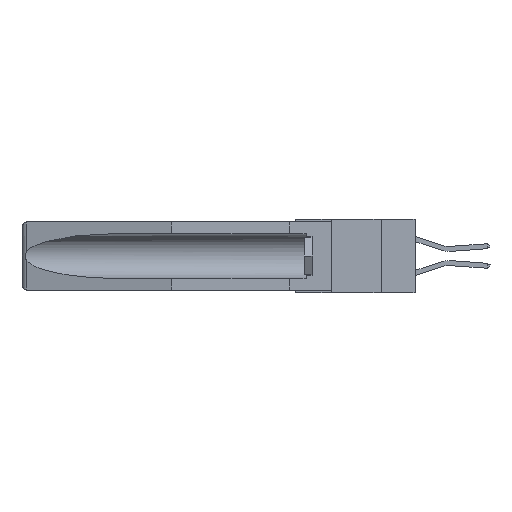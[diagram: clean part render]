
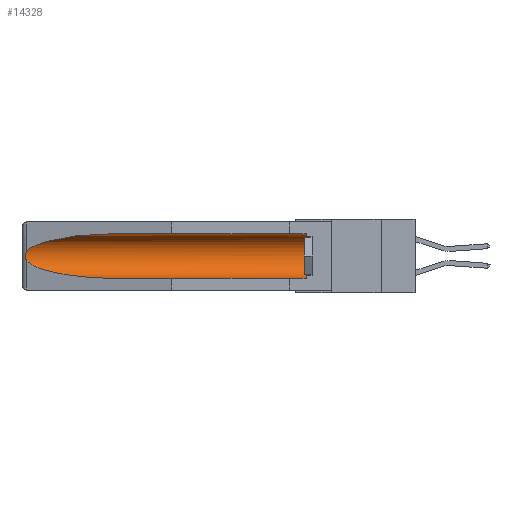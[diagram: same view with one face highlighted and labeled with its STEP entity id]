
A CAD part, left-side view. The second image highlights one B-rep face of the part: STEP entity #14328.
In plain terms, the highlighted cylindrical face has radius 2.857 mm (diameter 5.715 mm), a partial arc.
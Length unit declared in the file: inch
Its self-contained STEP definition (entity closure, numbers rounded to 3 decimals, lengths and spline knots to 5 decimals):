
#73 = B_SPLINE_CURVE_WITH_KNOTS ( 'NONE', 3,
 ( #18737, #18811, #20542, #18667, #11899, #1421, #1572, #13567, #13637, #15088 ),
 .UNSPECIFIED., .F., .F.,
 ( 4, 2, 2, 2, 4 ),
 ( 0., 0.00029, 0.00058, 0.00087, 0.00117 ),
 .UNSPECIFIED. ) ;
#281 = DIRECTION ( 'NONE',  ( 0., -1., 0. ) ) ;
#375 = CARTESIAN_POINT ( 'NONE',  ( 0.155, -0.30754, -0.059 ) ) ;
#984 = ORIENTED_EDGE ( 'NONE', *, *, #20544, .T. ) ;
#1224 = AXIS2_PLACEMENT_3D ( 'NONE', #21011, #281, #10690 ) ;
#1307 = CYLINDRICAL_SURFACE ( 'NONE', #9294, 0.1125 ) ;
#1421 = CARTESIAN_POINT ( 'NONE',  ( 0.2675, 1.53308, -0.17534 ) ) ;
#1572 = CARTESIAN_POINT ( 'NONE',  ( 0.2673, 1.53269, -0.17917 ) ) ;
#1577 = ORIENTED_EDGE ( 'NONE', *, *, #12082, .F. ) ;
#2076 = DIRECTION ( 'NONE',  ( 0., 0., 1. ) ) ;
#2409 = CARTESIAN_POINT ( 'NONE',  ( 0.21114, 1.30732, -0.284 ) ) ;
#3409 = CARTESIAN_POINT ( 'NONE',  ( 0.25451, 1.48313, -0.09465 ) ) ;
#4006 = CIRCLE ( 'NONE', #1224, 0.1125 ) ;
#6884 = EDGE_CURVE ( 'NONE', #11248, #16887, #19540, .T. ) ;
#6887 = CARTESIAN_POINT ( 'NONE',  ( 0.26537, 1.52718, -0.14972 ) ) ;
#6918 = ORIENTED_EDGE ( 'NONE', *, *, #6884, .T. ) ;
#7300 = CARTESIAN_POINT ( 'NONE',  ( 0.155, -0.30754, -0.1715 ) ) ;
#7549 = CARTESIAN_POINT ( 'NONE',  ( 0.155, 1.07973, -0.284 ) ) ;
#7848 = EDGE_LOOP ( 'NONE', ( #19603, #984, #9586, #1577, #12763, #6918 ) ) ;
#9294 = AXIS2_PLACEMENT_3D ( 'NONE', #7300, #10823, #2076 ) ;
#9586 = ORIENTED_EDGE ( 'NONE', *, *, #11202, .T. ) ;
#10166 =( BOUNDED_CURVE ( )  B_SPLINE_CURVE ( 3, ( #19640, #14554, #2409, #7549 ),
 .UNSPECIFIED., .F., .F. ) 
 B_SPLINE_CURVE_WITH_KNOTS ( ( 4, 4 ),
 ( 0.1948, 1.5708 ),
 .UNSPECIFIED. ) 
 CURVE ( )  GEOMETRIC_REPRESENTATION_ITEM ( )  RATIONAL_B_SPLINE_CURVE ( ( 1., 0.848, 0.848, 1. ) ) 
 REPRESENTATION_ITEM ( '' )  );
#10176 = CARTESIAN_POINT ( 'NONE',  ( 0.155, -0.30754, -0.284 ) ) ;
#10690 = DIRECTION ( 'NONE',  ( 0., 0., 1. ) ) ;
#10823 = DIRECTION ( 'NONE',  ( 0., 1., 0. ) ) ;
#10954 = CARTESIAN_POINT ( 'NONE',  ( 0.26537, 1.52718, -0.14972 ) ) ;
#11202 = EDGE_CURVE ( 'NONE', #21206, #16096, #10166, .T. ) ;
#11248 = VERTEX_POINT ( 'NONE', #21609 ) ;
#11439 = VERTEX_POINT ( 'NONE', #14534 ) ;
#11899 = CARTESIAN_POINT ( 'NONE',  ( 0.2675, 1.53308, -0.16763 ) ) ;
#12082 = EDGE_CURVE ( 'NONE', #11439, #16096, #14864, .T. ) ;
#12298 = VECTOR ( 'NONE', #19201, 39.37008 ) ;
#12425 = VECTOR ( 'NONE', #22234, 39.37008 ) ;
#12763 = ORIENTED_EDGE ( 'NONE', *, *, #13799, .T. ) ;
#13567 = CARTESIAN_POINT ( 'NONE',  ( 0.26655, 1.53094, -0.18657 ) ) ;
#13637 = CARTESIAN_POINT ( 'NONE',  ( 0.26597, 1.5296, -0.19026 ) ) ;
#13743 = CARTESIAN_POINT ( 'NONE',  ( 0.21114, 1.30732, -0.059 ) ) ;
#13799 = EDGE_CURVE ( 'NONE', #11439, #11248, #4006, .T. ) ;
#14328 = ADVANCED_FACE ( 'NONE', ( #15078 ), #1307, .F. ) ;
#14534 = CARTESIAN_POINT ( 'NONE',  ( 0.155, 0.126, -0.284 ) ) ;
#14554 = CARTESIAN_POINT ( 'NONE',  ( 0.25451, 1.48313, -0.24835 ) ) ;
#14864 = LINE ( 'NONE', #10176, #12425 ) ;
#15078 = FACE_OUTER_BOUND ( 'NONE', #7848, .T. ) ;
#15088 = CARTESIAN_POINT ( 'NONE',  ( 0.26537, 1.52718, -0.19328 ) ) ;
#15241 = CARTESIAN_POINT ( 'NONE',  ( 0.26537, 1.52718, -0.19328 ) ) ;
#15442 = CARTESIAN_POINT ( 'NONE',  ( 0.155, 1.07973, -0.059 ) ) ;
#16096 = VERTEX_POINT ( 'NONE', #16534 ) ;
#16534 = CARTESIAN_POINT ( 'NONE',  ( 0.155, 1.07973, -0.284 ) ) ;
#16887 = VERTEX_POINT ( 'NONE', #15442 ) ;
#18667 = CARTESIAN_POINT ( 'NONE',  ( 0.2673, 1.5327, -0.16383 ) ) ;
#18737 = CARTESIAN_POINT ( 'NONE',  ( 0.26537, 1.52718, -0.14972 ) ) ;
#18811 = CARTESIAN_POINT ( 'NONE',  ( 0.26597, 1.52961, -0.15275 ) ) ;
#18934 = VERTEX_POINT ( 'NONE', #10954 ) ;
#19201 = DIRECTION ( 'NONE',  ( 0., 1., 0. ) ) ;
#19316 = EDGE_CURVE ( 'NONE', #16887, #18934, #19427, .T. ) ;
#19427 =( BOUNDED_CURVE ( )  B_SPLINE_CURVE ( 3, ( #22308, #13743, #3409, #6887 ),
 .UNSPECIFIED., .F., .T. ) 
 B_SPLINE_CURVE_WITH_KNOTS ( ( 4, 4 ),
 ( 4.71239, 6.08839 ),
 .UNSPECIFIED. ) 
 CURVE ( )  GEOMETRIC_REPRESENTATION_ITEM ( )  RATIONAL_B_SPLINE_CURVE ( ( 1., 0.848, 0.848, 1. ) ) 
 REPRESENTATION_ITEM ( '' )  );
#19540 = LINE ( 'NONE', #375, #12298 ) ;
#19603 = ORIENTED_EDGE ( 'NONE', *, *, #19316, .T. ) ;
#19640 = CARTESIAN_POINT ( 'NONE',  ( 0.26537, 1.52718, -0.19328 ) ) ;
#20542 = CARTESIAN_POINT ( 'NONE',  ( 0.26654, 1.53092, -0.15636 ) ) ;
#20544 = EDGE_CURVE ( 'NONE', #18934, #21206, #73, .T. ) ;
#21011 = CARTESIAN_POINT ( 'NONE',  ( 0.155, 0.126, -0.1715 ) ) ;
#21206 = VERTEX_POINT ( 'NONE', #15241 ) ;
#21609 = CARTESIAN_POINT ( 'NONE',  ( 0.155, 0.126, -0.059 ) ) ;
#22234 = DIRECTION ( 'NONE',  ( 0., 1., 0. ) ) ;
#22308 = CARTESIAN_POINT ( 'NONE',  ( 0.155, 1.07973, -0.059 ) ) ;
